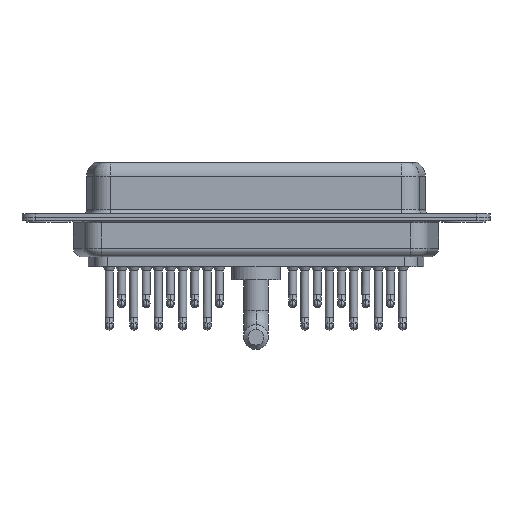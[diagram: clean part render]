
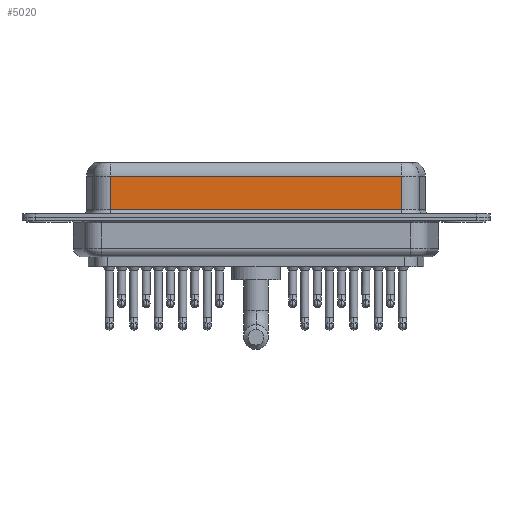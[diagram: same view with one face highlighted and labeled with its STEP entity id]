
A CAD part, front view. The second image highlights one B-rep face of the part: STEP entity #5020.
In plain terms, the highlighted planar face has unit normal (0, -1, 0).
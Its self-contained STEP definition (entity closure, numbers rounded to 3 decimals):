
#14 = DIRECTION ( 'NONE',  ( 0., 0., 1. ) ) ;
#196 = ORIENTED_EDGE ( 'NONE', *, *, #12997, .F. ) ;
#266 = DIRECTION ( 'NONE',  ( 0., 0., -1. ) ) ;
#1239 = VECTOR ( 'NONE', #9823, 1000. ) ;
#2364 = EDGE_CURVE ( 'NONE', #5018, #16850, #4288, .T. ) ;
#2435 = VECTOR ( 'NONE', #266, 1000. ) ;
#2788 = PLANE ( 'NONE',  #6523 ) ;
#3099 = FACE_OUTER_BOUND ( 'NONE', #9842, .T. ) ;
#3226 = ORIENTED_EDGE ( 'NONE', *, *, #2364, .T. ) ;
#4288 = LINE ( 'NONE', #18422, #11763 ) ;
#4625 = CARTESIAN_POINT ( 'NONE',  ( 7.013, -3.95, 0.9 ) ) ;
#5018 = VERTEX_POINT ( 'NONE', #17198 ) ;
#5020 = ADVANCED_FACE ( 'NONE', ( #3099 ), #2788, .F. ) ;
#6291 = CARTESIAN_POINT ( 'NONE',  ( 40.037, -3.95, 6.4 ) ) ;
#6523 = AXIS2_PLACEMENT_3D ( 'NONE', #15836, #17299, #14 ) ;
#7401 = CARTESIAN_POINT ( 'NONE',  ( 40.037, -3.95, 0.9 ) ) ;
#7827 = CARTESIAN_POINT ( 'NONE',  ( 40.037, -3.95, 0.9 ) ) ;
#8226 = LINE ( 'NONE', #7827, #1239 ) ;
#8372 = LINE ( 'NONE', #6291, #2435 ) ;
#8596 = VECTOR ( 'NONE', #15501, 1000. ) ;
#8775 = CARTESIAN_POINT ( 'NONE',  ( 40.037, -3.95, 4.65 ) ) ;
#9823 = DIRECTION ( 'NONE',  ( 1., 0., 0. ) ) ;
#9842 = EDGE_LOOP ( 'NONE', ( #196, #17602, #3226, #12531 ) ) ;
#11763 = VECTOR ( 'NONE', #18608, 1000. ) ;
#12201 = EDGE_CURVE ( 'NONE', #16850, #19647, #8226, .T. ) ;
#12531 = ORIENTED_EDGE ( 'NONE', *, *, #12201, .T. ) ;
#12997 = EDGE_CURVE ( 'NONE', #19509, #19647, #8372, .T. ) ;
#14134 = LINE ( 'NONE', #15596, #8596 ) ;
#15501 = DIRECTION ( 'NONE',  ( -1., 0., 0. ) ) ;
#15551 = EDGE_CURVE ( 'NONE', #19509, #5018, #14134, .T. ) ;
#15596 = CARTESIAN_POINT ( 'NONE',  ( 40.037, -3.95, 4.65 ) ) ;
#15836 = CARTESIAN_POINT ( 'NONE',  ( 40.037, -3.95, 6.4 ) ) ;
#16850 = VERTEX_POINT ( 'NONE', #4625 ) ;
#17198 = CARTESIAN_POINT ( 'NONE',  ( 7.013, -3.95, 4.65 ) ) ;
#17299 = DIRECTION ( 'NONE',  ( 0., 1., 0. ) ) ;
#17602 = ORIENTED_EDGE ( 'NONE', *, *, #15551, .T. ) ;
#18422 = CARTESIAN_POINT ( 'NONE',  ( 7.013, -3.95, 6.4 ) ) ;
#18608 = DIRECTION ( 'NONE',  ( 0., 0., -1. ) ) ;
#19509 = VERTEX_POINT ( 'NONE', #8775 ) ;
#19647 = VERTEX_POINT ( 'NONE', #7401 ) ;
